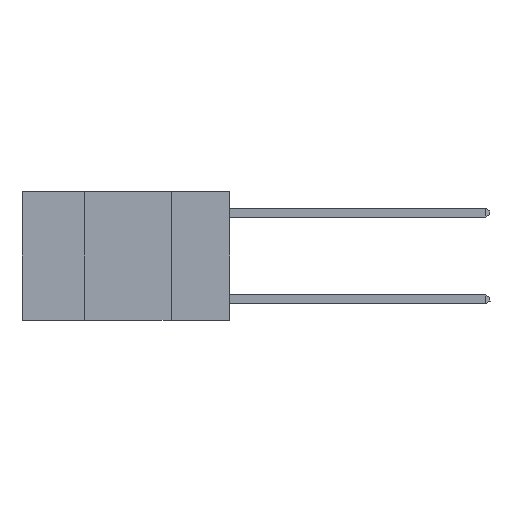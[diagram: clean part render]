
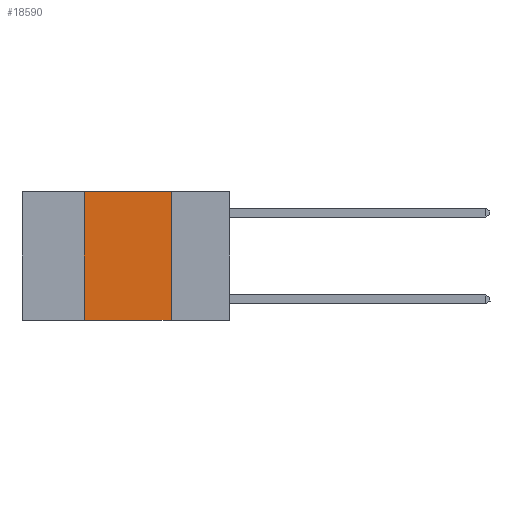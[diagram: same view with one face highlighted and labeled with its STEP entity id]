
A CAD part, left-side view. The second image highlights one B-rep face of the part: STEP entity #18590.
In plain terms, the highlighted planar face has unit normal (-1, 0, 0).
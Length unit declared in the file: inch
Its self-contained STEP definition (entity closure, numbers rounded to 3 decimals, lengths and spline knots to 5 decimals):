
#348 = DIRECTION ( 'NONE',  ( 0., 0., -1. ) ) ;
#535 = VECTOR ( 'NONE', #17655, 39.37008 ) ;
#1355 = DIRECTION ( 'NONE',  ( 0., 0., -1. ) ) ;
#1761 = VERTEX_POINT ( 'NONE', #2371 ) ;
#2371 = CARTESIAN_POINT ( 'NONE',  ( 0., 0.42, 0. ) ) ;
#3916 = FACE_OUTER_BOUND ( 'NONE', #15094, .T. ) ;
#4777 = LINE ( 'NONE', #25940, #9611 ) ;
#5000 = DIRECTION ( 'NONE',  ( 0., 0., 1. ) ) ;
#6110 = LINE ( 'NONE', #26605, #26002 ) ;
#7138 = ORIENTED_EDGE ( 'NONE', *, *, #13306, .F. ) ;
#7437 = CARTESIAN_POINT ( 'NONE',  ( 0., 0.42, -0.37 ) ) ;
#7672 = ORIENTED_EDGE ( 'NONE', *, *, #16106, .F. ) ;
#8338 = ORIENTED_EDGE ( 'NONE', *, *, #10047, .T. ) ;
#9611 = VECTOR ( 'NONE', #1355, 39.37008 ) ;
#9632 = CARTESIAN_POINT ( 'NONE',  ( 0., 0.17, 0. ) ) ;
#10047 = EDGE_CURVE ( 'NONE', #11879, #12615, #17094, .T. ) ;
#10733 = CARTESIAN_POINT ( 'NONE',  ( 0., 0.6, 0. ) ) ;
#11879 = VERTEX_POINT ( 'NONE', #7437 ) ;
#12447 = VECTOR ( 'NONE', #5000, 39.37008 ) ;
#12615 = VERTEX_POINT ( 'NONE', #13712 ) ;
#12806 = DIRECTION ( 'NONE',  ( 1., 0., 0. ) ) ;
#13306 = EDGE_CURVE ( 'NONE', #13321, #12615, #4777, .T. ) ;
#13321 = VERTEX_POINT ( 'NONE', #9632 ) ;
#13712 = CARTESIAN_POINT ( 'NONE',  ( 0., 0.17, -0.37 ) ) ;
#15094 = EDGE_LOOP ( 'NONE', ( #7138, #18088, #7672, #8338 ) ) ;
#15485 = AXIS2_PLACEMENT_3D ( 'NONE', #10733, #12806, #348 ) ;
#15598 = CARTESIAN_POINT ( 'NONE',  ( 0., 0.6, -0.37 ) ) ;
#15989 = LINE ( 'NONE', #23542, #12447 ) ;
#16106 = EDGE_CURVE ( 'NONE', #11879, #1761, #15989, .T. ) ;
#16470 = DIRECTION ( 'NONE',  ( 0., -1., 0. ) ) ;
#17094 = LINE ( 'NONE', #15598, #535 ) ;
#17655 = DIRECTION ( 'NONE',  ( 0., -1., 0. ) ) ;
#18088 = ORIENTED_EDGE ( 'NONE', *, *, #20849, .F. ) ;
#18590 = ADVANCED_FACE ( 'NONE', ( #3916 ), #23016, .F. ) ;
#20849 = EDGE_CURVE ( 'NONE', #1761, #13321, #6110, .T. ) ;
#23016 = PLANE ( 'NONE',  #15485 ) ;
#23542 = CARTESIAN_POINT ( 'NONE',  ( 0., 0.42, 0. ) ) ;
#25940 = CARTESIAN_POINT ( 'NONE',  ( 0., 0.17, 0. ) ) ;
#26002 = VECTOR ( 'NONE', #16470, 39.37008 ) ;
#26605 = CARTESIAN_POINT ( 'NONE',  ( 0., 0.6, 0. ) ) ;
